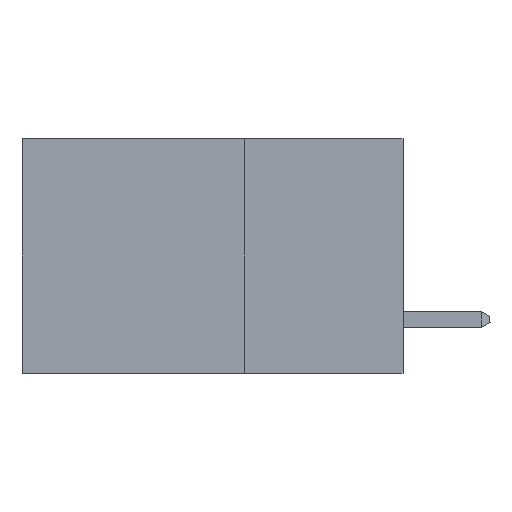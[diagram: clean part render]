
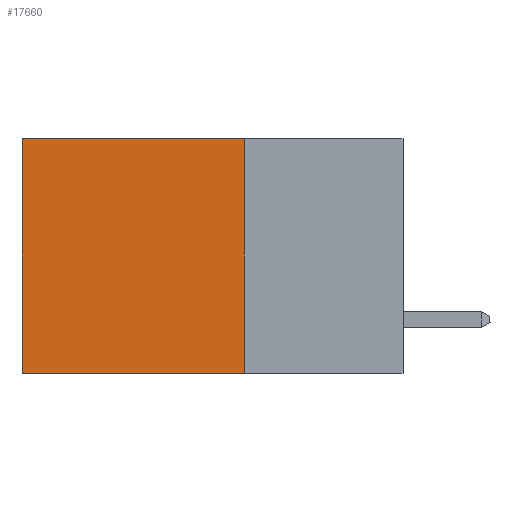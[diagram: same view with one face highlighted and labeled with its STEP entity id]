
A CAD part, left-side view. The second image highlights one B-rep face of the part: STEP entity #17660.
In plain terms, the highlighted planar face has unit normal (-1, 0, 0).
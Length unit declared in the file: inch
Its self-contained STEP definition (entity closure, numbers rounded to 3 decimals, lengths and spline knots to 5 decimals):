
#2011 = EDGE_CURVE ( 'NONE', #12587, #9936, #2194, .T. ) ;
#2194 = LINE ( 'NONE', #12032, #16315 ) ;
#2213 = DIRECTION ( 'NONE',  ( 0., 0., -1. ) ) ;
#2623 = LINE ( 'NONE', #6211, #24383 ) ;
#3213 = EDGE_CURVE ( 'NONE', #17476, #22528, #4918, .T. ) ;
#3666 = PLANE ( 'NONE',  #18871 ) ;
#4918 = LINE ( 'NONE', #21142, #19717 ) ;
#5282 = ORIENTED_EDGE ( 'NONE', *, *, #2011, .F. ) ;
#6211 = CARTESIAN_POINT ( 'NONE',  ( 0.2875, 0.25, 0. ) ) ;
#6361 = ORIENTED_EDGE ( 'NONE', *, *, #3213, .T. ) ;
#6372 = DIRECTION ( 'NONE',  ( 0., 1., 0. ) ) ;
#6427 = CARTESIAN_POINT ( 'NONE',  ( 0.2875, 0.6, 0. ) ) ;
#6944 = DIRECTION ( 'NONE',  ( 0., 0., -1. ) ) ;
#8398 = CARTESIAN_POINT ( 'NONE',  ( 0.2875, 0.25, -0.37 ) ) ;
#9936 = VERTEX_POINT ( 'NONE', #25895 ) ;
#10478 = CARTESIAN_POINT ( 'NONE',  ( 0.2875, 0.6, 0. ) ) ;
#10799 = EDGE_LOOP ( 'NONE', ( #11231, #5282, #15724, #6361 ) ) ;
#11231 = ORIENTED_EDGE ( 'NONE', *, *, #17925, .T. ) ;
#12032 = CARTESIAN_POINT ( 'NONE',  ( 0.2875, 0.25, -0.37 ) ) ;
#12587 = VERTEX_POINT ( 'NONE', #8398 ) ;
#14515 = DIRECTION ( 'NONE',  ( 0., 0., -1. ) ) ;
#15385 = VECTOR ( 'NONE', #14515, 39.37008 ) ;
#15724 = ORIENTED_EDGE ( 'NONE', *, *, #27143, .F. ) ;
#16315 = VECTOR ( 'NONE', #26739, 39.37008 ) ;
#17476 = VERTEX_POINT ( 'NONE', #17532 ) ;
#17532 = CARTESIAN_POINT ( 'NONE',  ( 0.2875, 0.25, 0. ) ) ;
#17660 = ADVANCED_FACE ( 'NONE', ( #25959 ), #3666, .F. ) ;
#17925 = EDGE_CURVE ( 'NONE', #22528, #9936, #23618, .T. ) ;
#18871 = AXIS2_PLACEMENT_3D ( 'NONE', #23820, #21613, #6944 ) ;
#19717 = VECTOR ( 'NONE', #6372, 39.37008 ) ;
#21142 = CARTESIAN_POINT ( 'NONE',  ( 0.2875, 0.25, 0. ) ) ;
#21613 = DIRECTION ( 'NONE',  ( 1., 0., 0. ) ) ;
#22528 = VERTEX_POINT ( 'NONE', #10478 ) ;
#23618 = LINE ( 'NONE', #6427, #15385 ) ;
#23820 = CARTESIAN_POINT ( 'NONE',  ( 0.2875, 0.25, 0. ) ) ;
#24383 = VECTOR ( 'NONE', #2213, 39.37008 ) ;
#25895 = CARTESIAN_POINT ( 'NONE',  ( 0.2875, 0.6, -0.37 ) ) ;
#25959 = FACE_OUTER_BOUND ( 'NONE', #10799, .T. ) ;
#26739 = DIRECTION ( 'NONE',  ( 0., 1., 0. ) ) ;
#27143 = EDGE_CURVE ( 'NONE', #17476, #12587, #2623, .T. ) ;
